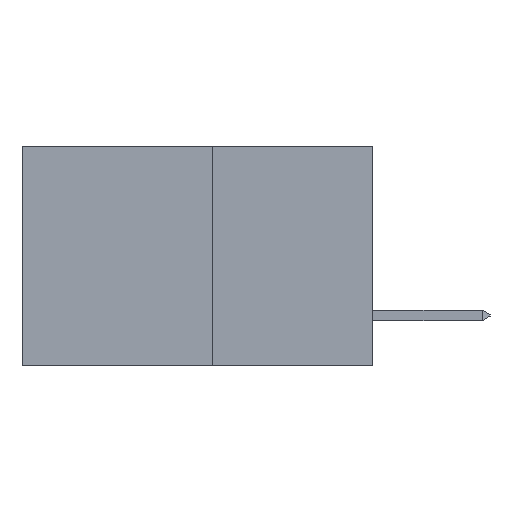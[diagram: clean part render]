
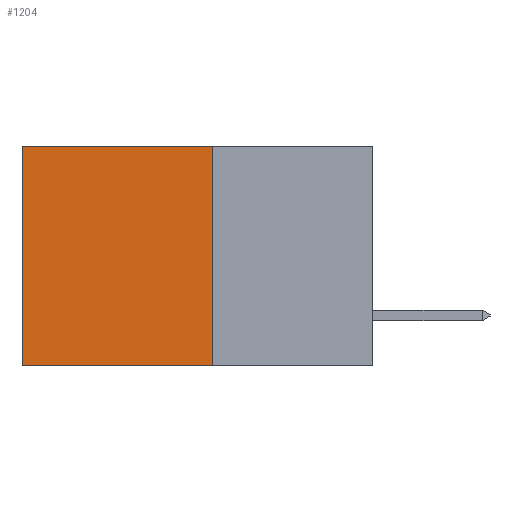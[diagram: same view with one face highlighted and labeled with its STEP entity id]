
A CAD part, left-side view. The second image highlights one B-rep face of the part: STEP entity #1204.
In plain terms, the highlighted planar face has unit normal (-1, 0, 0).
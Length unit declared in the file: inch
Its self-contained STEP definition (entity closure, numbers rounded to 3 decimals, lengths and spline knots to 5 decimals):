
#427 = LINE ( 'NONE', #13682, #15235 ) ;
#1204 = ADVANCED_FACE ( 'NONE', ( #11246 ), #11568, .F. ) ;
#1361 = DIRECTION ( 'NONE',  ( 0., 0., -1. ) ) ;
#1415 = DIRECTION ( 'NONE',  ( 1., 0., 0. ) ) ;
#2197 = LINE ( 'NONE', #14719, #11856 ) ;
#3098 = VERTEX_POINT ( 'NONE', #6923 ) ;
#3329 = CARTESIAN_POINT ( 'NONE',  ( 0.277, 0.27, 0. ) ) ;
#4166 = VECTOR ( 'NONE', #7041, 39.37008 ) ;
#4710 = CARTESIAN_POINT ( 'NONE',  ( 0.277, 0.27, 0. ) ) ;
#4820 = EDGE_CURVE ( 'NONE', #11703, #3098, #427, .T. ) ;
#5292 = DIRECTION ( 'NONE',  ( 0., 0., -1. ) ) ;
#6124 = VECTOR ( 'NONE', #6951, 39.37008 ) ;
#6506 = DIRECTION ( 'NONE',  ( 0., 0., -1. ) ) ;
#6923 = CARTESIAN_POINT ( 'NONE',  ( 0.277, 0.59, -0.37 ) ) ;
#6936 = CARTESIAN_POINT ( 'NONE',  ( 0.277, 0.59, 0. ) ) ;
#6951 = DIRECTION ( 'NONE',  ( 0., 1., 0. ) ) ;
#7041 = DIRECTION ( 'NONE',  ( 0., 1., 0. ) ) ;
#8519 = VERTEX_POINT ( 'NONE', #4710 ) ;
#8537 = VERTEX_POINT ( 'NONE', #14194 ) ;
#8684 = AXIS2_PLACEMENT_3D ( 'NONE', #11524, #1415, #1361 ) ;
#9034 = ORIENTED_EDGE ( 'NONE', *, *, #4820, .T. ) ;
#9318 = EDGE_CURVE ( 'NONE', #8519, #8537, #2197, .T. ) ;
#9782 = EDGE_LOOP ( 'NONE', ( #9034, #12156, #12888, #12725 ) ) ;
#11246 = FACE_OUTER_BOUND ( 'NONE', #9782, .T. ) ;
#11524 = CARTESIAN_POINT ( 'NONE',  ( 0.277, 0.27, -0.37 ) ) ;
#11568 = PLANE ( 'NONE',  #8684 ) ;
#11703 = VERTEX_POINT ( 'NONE', #6936 ) ;
#11856 = VECTOR ( 'NONE', #6506, 39.37008 ) ;
#12047 = LINE ( 'NONE', #15132, #6124 ) ;
#12156 = ORIENTED_EDGE ( 'NONE', *, *, #13090, .F. ) ;
#12725 = ORIENTED_EDGE ( 'NONE', *, *, #14615, .T. ) ;
#12888 = ORIENTED_EDGE ( 'NONE', *, *, #9318, .F. ) ;
#13090 = EDGE_CURVE ( 'NONE', #8537, #3098, #12047, .T. ) ;
#13681 = LINE ( 'NONE', #3329, #4166 ) ;
#13682 = CARTESIAN_POINT ( 'NONE',  ( 0.277, 0.59, -0.37 ) ) ;
#14194 = CARTESIAN_POINT ( 'NONE',  ( 0.277, 0.27, -0.37 ) ) ;
#14615 = EDGE_CURVE ( 'NONE', #8519, #11703, #13681, .T. ) ;
#14719 = CARTESIAN_POINT ( 'NONE',  ( 0.277, 0.27, -0.37 ) ) ;
#15132 = CARTESIAN_POINT ( 'NONE',  ( 0.277, 0.27, -0.37 ) ) ;
#15235 = VECTOR ( 'NONE', #5292, 39.37008 ) ;
